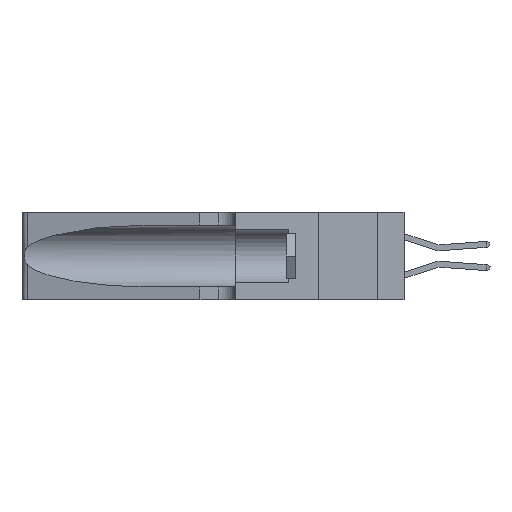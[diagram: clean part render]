
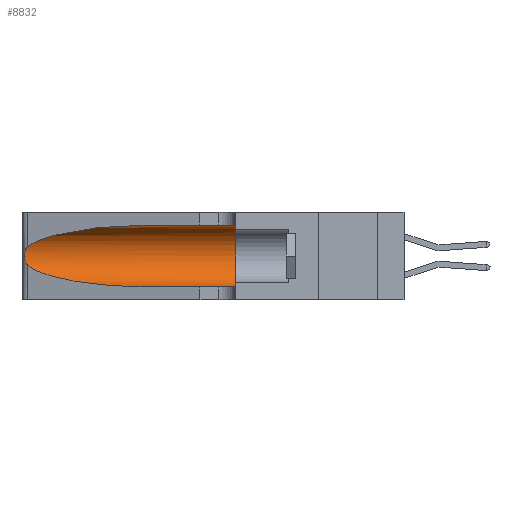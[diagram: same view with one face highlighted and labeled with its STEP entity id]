
A CAD part, left-side view. The second image highlights one B-rep face of the part: STEP entity #8832.
In plain terms, the highlighted cylindrical face has radius 3.308 mm (diameter 6.617 mm), a partial arc.
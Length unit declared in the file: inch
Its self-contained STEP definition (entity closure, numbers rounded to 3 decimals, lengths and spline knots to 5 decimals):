
#54 = CARTESIAN_POINT ( 'NONE',  ( 0.1305, 1.61858, 0.185 ) ) ;
#144 = DIRECTION ( 'NONE',  ( 0., -1., 0. ) ) ;
#393 = EDGE_CURVE ( 'NONE', #625, #23759, #1854, .T. ) ;
#625 = VERTEX_POINT ( 'NONE', #2886 ) ;
#723 = EDGE_CURVE ( 'NONE', #10495, #16219, #19017, .T. ) ;
#1674 = AXIS2_PLACEMENT_3D ( 'NONE', #4981, #19137, #7043 ) ;
#1753 = CARTESIAN_POINT ( 'NONE',  ( 0.26075, 1.23896, 0.178 ) ) ;
#1854 = LINE ( 'NONE', #16795, #12091 ) ;
#2512 = CYLINDRICAL_SURFACE ( 'NONE', #12548, 0.13025 ) ;
#2590 = CIRCLE ( 'NONE', #1674, 0.13025 ) ;
#2886 = CARTESIAN_POINT ( 'NONE',  ( 0.1305, 0.72297, 0.05475 ) ) ;
#3839 = CARTESIAN_POINT ( 'NONE',  ( 0.25856, 1.23593, 0.16098 ) ) ;
#4060 = CARTESIAN_POINT ( 'NONE',  ( 0.25487, 1.22718, 0.14631 ) ) ;
#4202 = DIRECTION ( 'NONE',  ( 0., -1., 0. ) ) ;
#4895 =( BOUNDED_CURVE ( )  B_SPLINE_CURVE ( 3, ( #4060, #6122, #20276, #8179 ),
 .UNSPECIFIED., .F., .T. ) 
 B_SPLINE_CURVE_WITH_KNOTS ( ( 4, 4 ),
 ( 3.44316, 4.71239 ),
 .UNSPECIFIED. ) 
 CURVE ( )  GEOMETRIC_REPRESENTATION_ITEM ( )  RATIONAL_B_SPLINE_CURVE ( ( 1., 0.87, 0.87, 1. ) ) 
 REPRESENTATION_ITEM ( '' )  );
#4981 = CARTESIAN_POINT ( 'NONE',  ( 0.1305, 0.35, 0.185 ) ) ;
#5918 = CARTESIAN_POINT ( 'NONE',  ( 0.25639, 1.23186, 0.15144 ) ) ;
#6122 = CARTESIAN_POINT ( 'NONE',  ( 0.2373, 1.15595, 0.08982 ) ) ;
#6757 = ORIENTED_EDGE ( 'NONE', *, *, #8171, .T. ) ;
#7043 = DIRECTION ( 'NONE',  ( 0., 0., 1. ) ) ;
#7658 = VERTEX_POINT ( 'NONE', #18788 ) ;
#7784 = ORIENTED_EDGE ( 'NONE', *, *, #14016, .T. ) ;
#7967 = CARTESIAN_POINT ( 'NONE',  ( 0.25487, 1.22718, 0.14631 ) ) ;
#8171 = EDGE_CURVE ( 'NONE', #10613, #625, #4895, .T. ) ;
#8179 = CARTESIAN_POINT ( 'NONE',  ( 0.1305, 0.72297, 0.05475 ) ) ;
#8832 = ADVANCED_FACE ( 'NONE', ( #19361 ), #2512, .F. ) ;
#8859 = EDGE_CURVE ( 'NONE', #10495, #7658, #13358, .T. ) ;
#9520 = ORIENTED_EDGE ( 'NONE', *, *, #22012, .F. ) ;
#9939 = CARTESIAN_POINT ( 'NONE',  ( 0.25639, 1.23184, 0.21858 ) ) ;
#10063 = ORIENTED_EDGE ( 'NONE', *, *, #393, .T. ) ;
#10495 = VERTEX_POINT ( 'NONE', #12802 ) ;
#10613 = VERTEX_POINT ( 'NONE', #25306 ) ;
#11870 = CARTESIAN_POINT ( 'NONE',  ( 0.25555, 1.22994, 0.2215 ) ) ;
#11955 = CARTESIAN_POINT ( 'NONE',  ( 0.25854, 1.2359, 0.20912 ) ) ;
#12091 = VECTOR ( 'NONE', #24003, 39.37008 ) ;
#12381 = B_SPLINE_CURVE_WITH_KNOTS ( 'NONE', 3,
 ( #15885, #11870, #9939, #24040, #11955, #26020, #13965, #1753, #15971, #3839, #18046, #5918, #20065, #7967 ),
 .UNSPECIFIED., .F., .F.,
 ( 4, 2, 2, 2, 2, 2, 4 ),
 ( 0., 0.00027, 0.00053, 0.00107, 0.0016, 0.00187, 0.00214 ),
 .UNSPECIFIED. ) ;
#12548 = AXIS2_PLACEMENT_3D ( 'NONE', #54, #4202, #18391 ) ;
#12802 = CARTESIAN_POINT ( 'NONE',  ( 0.1305, 0.72297, 0.31525 ) ) ;
#13358 = LINE ( 'NONE', #24461, #23460 ) ;
#13957 = CARTESIAN_POINT ( 'NONE',  ( 0.1305, 0.72297, 0.31525 ) ) ;
#13965 = CARTESIAN_POINT ( 'NONE',  ( 0.26075, 1.23896, 0.19203 ) ) ;
#14016 = EDGE_CURVE ( 'NONE', #16219, #10613, #12381, .T. ) ;
#14377 = CARTESIAN_POINT ( 'NONE',  ( 0.25487, 1.22718, 0.22369 ) ) ;
#14684 = CARTESIAN_POINT ( 'NONE',  ( 0.18966, 0.96281, 0.31525 ) ) ;
#15542 = CARTESIAN_POINT ( 'NONE',  ( 0.25487, 1.22718, 0.22369 ) ) ;
#15885 = CARTESIAN_POINT ( 'NONE',  ( 0.25487, 1.22718, 0.22369 ) ) ;
#15971 = CARTESIAN_POINT ( 'NONE',  ( 0.26017, 1.23833, 0.17102 ) ) ;
#16219 = VERTEX_POINT ( 'NONE', #15542 ) ;
#16795 = CARTESIAN_POINT ( 'NONE',  ( 0.1305, 1.61858, 0.05475 ) ) ;
#18046 = CARTESIAN_POINT ( 'NONE',  ( 0.25789, 1.23486, 0.15765 ) ) ;
#18391 = DIRECTION ( 'NONE',  ( 0., 0., -1. ) ) ;
#18788 = CARTESIAN_POINT ( 'NONE',  ( 0.1305, 0.35, 0.31525 ) ) ;
#19017 =( BOUNDED_CURVE ( )  B_SPLINE_CURVE ( 3, ( #13957, #14684, #23940, #14377 ),
 .UNSPECIFIED., .F., .F. ) 
 B_SPLINE_CURVE_WITH_KNOTS ( ( 4, 4 ),
 ( 1.5708, 2.84003 ),
 .UNSPECIFIED. ) 
 CURVE ( )  GEOMETRIC_REPRESENTATION_ITEM ( )  RATIONAL_B_SPLINE_CURVE ( ( 1., 0.87, 0.87, 1. ) ) 
 REPRESENTATION_ITEM ( '' )  );
#19137 = DIRECTION ( 'NONE',  ( 0., 1., 0. ) ) ;
#19361 = FACE_OUTER_BOUND ( 'NONE', #21930, .T. ) ;
#20065 = CARTESIAN_POINT ( 'NONE',  ( 0.25555, 1.22993, 0.14849 ) ) ;
#20276 = CARTESIAN_POINT ( 'NONE',  ( 0.18966, 0.96281, 0.05475 ) ) ;
#20986 = ORIENTED_EDGE ( 'NONE', *, *, #723, .T. ) ;
#21930 = EDGE_LOOP ( 'NONE', ( #20986, #7784, #6757, #10063, #9520, #25559 ) ) ;
#22012 = EDGE_CURVE ( 'NONE', #7658, #23759, #2590, .T. ) ;
#22332 = CARTESIAN_POINT ( 'NONE',  ( 0.1305, 0.35, 0.05475 ) ) ;
#23460 = VECTOR ( 'NONE', #144, 39.37008 ) ;
#23759 = VERTEX_POINT ( 'NONE', #22332 ) ;
#23940 = CARTESIAN_POINT ( 'NONE',  ( 0.2373, 1.15595, 0.28018 ) ) ;
#24003 = DIRECTION ( 'NONE',  ( 0., -1., 0. ) ) ;
#24040 = CARTESIAN_POINT ( 'NONE',  ( 0.25787, 1.23484, 0.2124 ) ) ;
#24461 = CARTESIAN_POINT ( 'NONE',  ( 0.1305, 1.61858, 0.31525 ) ) ;
#25306 = CARTESIAN_POINT ( 'NONE',  ( 0.25487, 1.22718, 0.14631 ) ) ;
#25559 = ORIENTED_EDGE ( 'NONE', *, *, #8859, .F. ) ;
#26020 = CARTESIAN_POINT ( 'NONE',  ( 0.26018, 1.23835, 0.19895 ) ) ;
